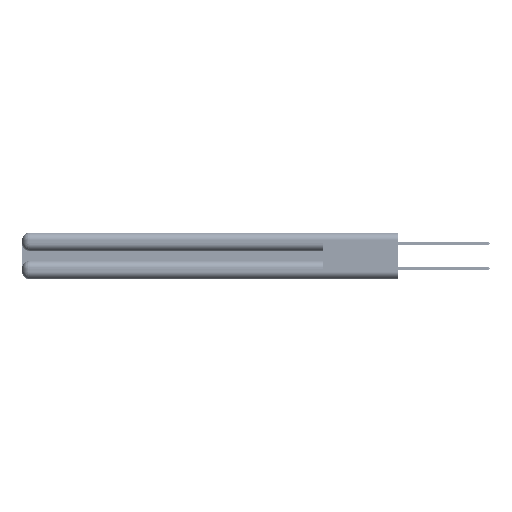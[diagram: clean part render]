
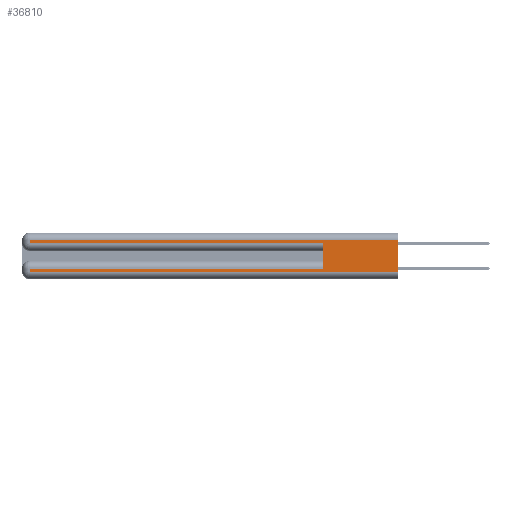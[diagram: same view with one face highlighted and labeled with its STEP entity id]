
A CAD part, left-side view. The second image highlights one B-rep face of the part: STEP entity #36810.
In plain terms, the highlighted planar face has unit normal (-1, 0, 0).
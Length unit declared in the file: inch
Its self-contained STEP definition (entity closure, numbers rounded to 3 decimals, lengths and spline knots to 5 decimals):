
#286 = CARTESIAN_POINT ( 'NONE',  ( 0., 2.94, 0.285 ) ) ;
#383 = ORIENTED_EDGE ( 'NONE', *, *, #32631, .T. ) ;
#2270 = CARTESIAN_POINT ( 'NONE',  ( 0., 0., 0.31 ) ) ;
#4270 = CARTESIAN_POINT ( 'NONE',  ( 0., 0., 0.285 ) ) ;
#4531 = DIRECTION ( 'NONE',  ( 0., 0., -1. ) ) ;
#5758 = EDGE_CURVE ( 'NONE', #31106, #44356, #31450, .T. ) ;
#5766 = DIRECTION ( 'NONE',  ( 0., -1., 0. ) ) ;
#10024 = CARTESIAN_POINT ( 'NONE',  ( 0., 0., 0.31 ) ) ;
#10542 = DIRECTION ( 'NONE',  ( 0., 1., 0. ) ) ;
#10776 = CARTESIAN_POINT ( 'NONE',  ( 0., 0., 0.37 ) ) ;
#12460 = EDGE_CURVE ( 'NONE', #47753, #43689, #41574, .T. ) ;
#15028 = DIRECTION ( 'NONE',  ( 1., 0., 0. ) ) ;
#15497 = AXIS2_PLACEMENT_3D ( 'NONE', #10776, #15028, #19085 ) ;
#15688 = VECTOR ( 'NONE', #50914, 39.37008 ) ;
#15842 = VECTOR ( 'NONE', #4531, 39.37008 ) ;
#17235 = EDGE_CURVE ( 'NONE', #43689, #48688, #22799, .T. ) ;
#17379 = CARTESIAN_POINT ( 'NONE',  ( 0., 0., 0.06 ) ) ;
#18190 = CARTESIAN_POINT ( 'NONE',  ( 0., 2.94, 0.31 ) ) ;
#19085 = DIRECTION ( 'NONE',  ( 0., 0., -1. ) ) ;
#19124 = ORIENTED_EDGE ( 'NONE', *, *, #23903, .T. ) ;
#19438 = PLANE ( 'NONE',  #15497 ) ;
#19448 = CARTESIAN_POINT ( 'NONE',  ( 0., 2.94, 0.37 ) ) ;
#19982 = LINE ( 'NONE', #19448, #51062 ) ;
#22799 = LINE ( 'NONE', #50199, #51312 ) ;
#23903 = EDGE_CURVE ( 'NONE', #26857, #29342, #19982, .T. ) ;
#24452 = ORIENTED_EDGE ( 'NONE', *, *, #31867, .T. ) ;
#26857 = VERTEX_POINT ( 'NONE', #18190 ) ;
#27572 = ORIENTED_EDGE ( 'NONE', *, *, #33023, .T. ) ;
#27602 = VECTOR ( 'NONE', #48718, 39.37008 ) ;
#28306 = EDGE_CURVE ( 'NONE', #36589, #48688, #46862, .T. ) ;
#29342 = VERTEX_POINT ( 'NONE', #286 ) ;
#31106 = VERTEX_POINT ( 'NONE', #41264 ) ;
#31450 = LINE ( 'NONE', #46839, #15688 ) ;
#31867 = EDGE_CURVE ( 'NONE', #36589, #26857, #52398, .T. ) ;
#32114 = ORIENTED_EDGE ( 'NONE', *, *, #5758, .F. ) ;
#32147 = CARTESIAN_POINT ( 'NONE',  ( 0., 0., 0.37 ) ) ;
#32606 = VECTOR ( 'NONE', #51681, 39.37008 ) ;
#32631 = EDGE_CURVE ( 'NONE', #29342, #44356, #52301, .T. ) ;
#33023 = EDGE_CURVE ( 'NONE', #31106, #47753, #42746, .T. ) ;
#34146 = CARTESIAN_POINT ( 'NONE',  ( 0., 0.6, 0.285 ) ) ;
#34189 = CARTESIAN_POINT ( 'NONE',  ( 0., 2.94, 0.06 ) ) ;
#34292 = FACE_OUTER_BOUND ( 'NONE', #40716, .T. ) ;
#35378 = CARTESIAN_POINT ( 'NONE',  ( 0., 0., 0.085 ) ) ;
#35713 = DIRECTION ( 'NONE',  ( 0., 0., -1. ) ) ;
#36589 = VERTEX_POINT ( 'NONE', #2270 ) ;
#36810 = ADVANCED_FACE ( 'NONE', ( #34292 ), #19438, .F. ) ;
#37852 = ORIENTED_EDGE ( 'NONE', *, *, #12460, .T. ) ;
#40444 = CARTESIAN_POINT ( 'NONE',  ( 0., 2.94, 0.37 ) ) ;
#40488 = CARTESIAN_POINT ( 'NONE',  ( 0., 2.94, 0.085 ) ) ;
#40716 = EDGE_LOOP ( 'NONE', ( #48620, #24452, #19124, #383, #32114, #27572, #37852, #42434 ) ) ;
#41264 = CARTESIAN_POINT ( 'NONE',  ( 0., 0.6, 0.085 ) ) ;
#41574 = LINE ( 'NONE', #40444, #41744 ) ;
#41744 = VECTOR ( 'NONE', #44472, 39.37008 ) ;
#42434 = ORIENTED_EDGE ( 'NONE', *, *, #17235, .T. ) ;
#42746 = LINE ( 'NONE', #35378, #32606 ) ;
#43689 = VERTEX_POINT ( 'NONE', #34189 ) ;
#44356 = VERTEX_POINT ( 'NONE', #34146 ) ;
#44472 = DIRECTION ( 'NONE',  ( 0., 0., -1. ) ) ;
#46839 = CARTESIAN_POINT ( 'NONE',  ( 0., 0.6, 0.145 ) ) ;
#46862 = LINE ( 'NONE', #32147, #15842 ) ;
#47753 = VERTEX_POINT ( 'NONE', #40488 ) ;
#48583 = VECTOR ( 'NONE', #10542, 39.37008 ) ;
#48620 = ORIENTED_EDGE ( 'NONE', *, *, #28306, .F. ) ;
#48688 = VERTEX_POINT ( 'NONE', #17379 ) ;
#48718 = DIRECTION ( 'NONE',  ( 0., -1., 0. ) ) ;
#50199 = CARTESIAN_POINT ( 'NONE',  ( 0., 0., 0.06 ) ) ;
#50914 = DIRECTION ( 'NONE',  ( 0., 0., 1. ) ) ;
#51062 = VECTOR ( 'NONE', #35713, 39.37008 ) ;
#51312 = VECTOR ( 'NONE', #5766, 39.37008 ) ;
#51681 = DIRECTION ( 'NONE',  ( 0., 1., 0. ) ) ;
#52301 = LINE ( 'NONE', #4270, #27602 ) ;
#52398 = LINE ( 'NONE', #10024, #48583 ) ;
